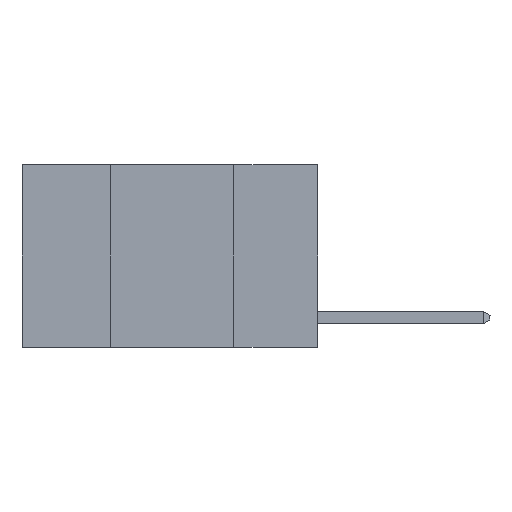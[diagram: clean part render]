
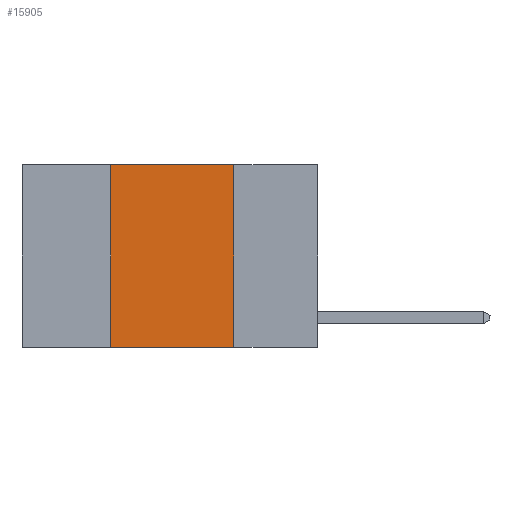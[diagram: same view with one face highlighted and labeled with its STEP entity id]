
A CAD part, left-side view. The second image highlights one B-rep face of the part: STEP entity #15905.
In plain terms, the highlighted planar face has unit normal (-1, 0, 0).
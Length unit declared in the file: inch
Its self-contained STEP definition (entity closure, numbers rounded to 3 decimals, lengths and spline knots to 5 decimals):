
#837 = CARTESIAN_POINT ( 'NONE',  ( 0., 0.42, 0. ) ) ;
#1079 = ORIENTED_EDGE ( 'NONE', *, *, #4374, .T. ) ;
#1175 = LINE ( 'NONE', #15855, #1614 ) ;
#1323 = LINE ( 'NONE', #4694, #21344 ) ;
#1614 = VECTOR ( 'NONE', #23162, 39.37008 ) ;
#1658 = ORIENTED_EDGE ( 'NONE', *, *, #15514, .F. ) ;
#3293 = VERTEX_POINT ( 'NONE', #17361 ) ;
#4374 = EDGE_CURVE ( 'NONE', #3293, #15117, #4591, .T. ) ;
#4591 = LINE ( 'NONE', #10359, #13821 ) ;
#4694 = CARTESIAN_POINT ( 'NONE',  ( 0., 0.6, 0. ) ) ;
#6199 = AXIS2_PLACEMENT_3D ( 'NONE', #14714, #22384, #14952 ) ;
#6392 = LINE ( 'NONE', #23127, #17043 ) ;
#6962 = CARTESIAN_POINT ( 'NONE',  ( 0., 0.17, -0.37 ) ) ;
#7567 = PLANE ( 'NONE',  #6199 ) ;
#7870 = EDGE_CURVE ( 'NONE', #19162, #23716, #1323, .T. ) ;
#10359 = CARTESIAN_POINT ( 'NONE',  ( 0., 0.6, -0.37 ) ) ;
#10560 = ORIENTED_EDGE ( 'NONE', *, *, #17554, .F. ) ;
#12509 = ORIENTED_EDGE ( 'NONE', *, *, #7870, .F. ) ;
#12530 = DIRECTION ( 'NONE',  ( 0., -1., 0. ) ) ;
#13776 = DIRECTION ( 'NONE',  ( 0., 0., 1. ) ) ;
#13821 = VECTOR ( 'NONE', #15553, 39.37008 ) ;
#14714 = CARTESIAN_POINT ( 'NONE',  ( 0., 0.6, 0. ) ) ;
#14840 = EDGE_LOOP ( 'NONE', ( #1658, #12509, #10560, #1079 ) ) ;
#14952 = DIRECTION ( 'NONE',  ( 0., 0., -1. ) ) ;
#15058 = FACE_OUTER_BOUND ( 'NONE', #14840, .T. ) ;
#15117 = VERTEX_POINT ( 'NONE', #6962 ) ;
#15514 = EDGE_CURVE ( 'NONE', #23716, #15117, #1175, .T. ) ;
#15553 = DIRECTION ( 'NONE',  ( 0., -1., 0. ) ) ;
#15855 = CARTESIAN_POINT ( 'NONE',  ( 0., 0.17, 0. ) ) ;
#15905 = ADVANCED_FACE ( 'NONE', ( #15058 ), #7567, .F. ) ;
#17043 = VECTOR ( 'NONE', #13776, 39.37008 ) ;
#17361 = CARTESIAN_POINT ( 'NONE',  ( 0., 0.42, -0.37 ) ) ;
#17554 = EDGE_CURVE ( 'NONE', #3293, #19162, #6392, .T. ) ;
#19162 = VERTEX_POINT ( 'NONE', #837 ) ;
#21344 = VECTOR ( 'NONE', #12530, 39.37008 ) ;
#22384 = DIRECTION ( 'NONE',  ( 1., 0., 0. ) ) ;
#23127 = CARTESIAN_POINT ( 'NONE',  ( 0., 0.42, 0. ) ) ;
#23162 = DIRECTION ( 'NONE',  ( 0., 0., -1. ) ) ;
#23235 = CARTESIAN_POINT ( 'NONE',  ( 0., 0.17, 0. ) ) ;
#23716 = VERTEX_POINT ( 'NONE', #23235 ) ;
